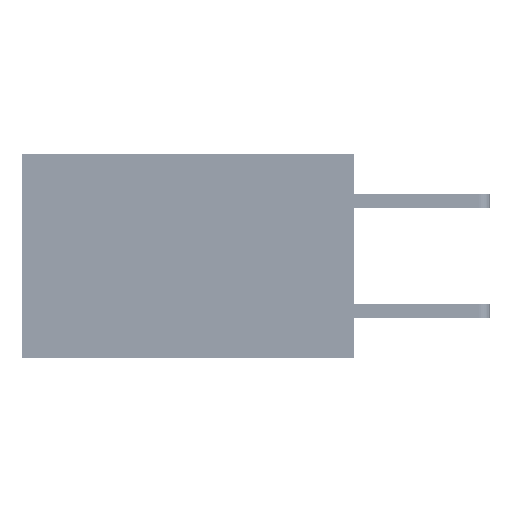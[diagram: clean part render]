
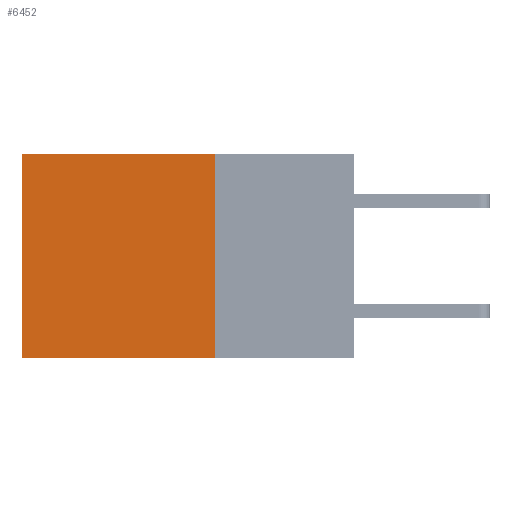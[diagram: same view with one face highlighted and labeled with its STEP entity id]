
A CAD part, left-side view. The second image highlights one B-rep face of the part: STEP entity #6452.
In plain terms, the highlighted planar face has unit normal (-1, 0, 0).
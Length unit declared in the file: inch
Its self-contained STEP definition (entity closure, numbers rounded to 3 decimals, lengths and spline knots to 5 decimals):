
#1216 = DIRECTION ( 'NONE',  ( 0., 0., -1. ) ) ;
#2729 = CARTESIAN_POINT ( 'NONE',  ( 0.2875, 0.25, -0.37 ) ) ;
#2798 = ORIENTED_EDGE ( 'NONE', *, *, #7453, .T. ) ;
#2869 = DIRECTION ( 'NONE',  ( 0., 1., 0. ) ) ;
#5285 = ORIENTED_EDGE ( 'NONE', *, *, #21799, .T. ) ;
#6452 = ADVANCED_FACE ( 'NONE', ( #37679 ), #11612, .F. ) ;
#7200 = VERTEX_POINT ( 'NONE', #37165 ) ;
#7284 = AXIS2_PLACEMENT_3D ( 'NONE', #11478, #27236, #24142 ) ;
#7453 = EDGE_CURVE ( 'NONE', #7200, #17033, #25143, .T. ) ;
#8992 = CARTESIAN_POINT ( 'NONE',  ( 0.2875, 0.6, 0. ) ) ;
#9237 = CARTESIAN_POINT ( 'NONE',  ( 0.2875, 0.25, -0.37 ) ) ;
#9628 = VECTOR ( 'NONE', #20769, 39.37008 ) ;
#10215 = VECTOR ( 'NONE', #2869, 39.37008 ) ;
#11478 = CARTESIAN_POINT ( 'NONE',  ( 0.2875, 0.25, 0. ) ) ;
#11612 = PLANE ( 'NONE',  #7284 ) ;
#14807 = VECTOR ( 'NONE', #26181, 39.37008 ) ;
#15288 = EDGE_CURVE ( 'NONE', #7200, #36131, #28277, .T. ) ;
#17033 = VERTEX_POINT ( 'NONE', #8992 ) ;
#20694 = CARTESIAN_POINT ( 'NONE',  ( 0.2875, 0.6, -0.37 ) ) ;
#20769 = DIRECTION ( 'NONE',  ( 0., 1., 0. ) ) ;
#20928 = ORIENTED_EDGE ( 'NONE', *, *, #15288, .F. ) ;
#20970 = EDGE_LOOP ( 'NONE', ( #5285, #35412, #20928, #2798 ) ) ;
#21799 = EDGE_CURVE ( 'NONE', #17033, #30639, #35271, .T. ) ;
#24142 = DIRECTION ( 'NONE',  ( 0., 0., -1. ) ) ;
#25143 = LINE ( 'NONE', #36661, #9628 ) ;
#26181 = DIRECTION ( 'NONE',  ( 0., 0., -1. ) ) ;
#27236 = DIRECTION ( 'NONE',  ( 1., 0., 0. ) ) ;
#28277 = LINE ( 'NONE', #29277, #14807 ) ;
#28812 = VECTOR ( 'NONE', #1216, 39.37008 ) ;
#29277 = CARTESIAN_POINT ( 'NONE',  ( 0.2875, 0.25, 0. ) ) ;
#30639 = VERTEX_POINT ( 'NONE', #20694 ) ;
#30764 = EDGE_CURVE ( 'NONE', #36131, #30639, #34166, .T. ) ;
#33286 = CARTESIAN_POINT ( 'NONE',  ( 0.2875, 0.6, 0. ) ) ;
#34166 = LINE ( 'NONE', #2729, #10215 ) ;
#35271 = LINE ( 'NONE', #33286, #28812 ) ;
#35412 = ORIENTED_EDGE ( 'NONE', *, *, #30764, .F. ) ;
#36131 = VERTEX_POINT ( 'NONE', #9237 ) ;
#36661 = CARTESIAN_POINT ( 'NONE',  ( 0.2875, 0.25, 0. ) ) ;
#37165 = CARTESIAN_POINT ( 'NONE',  ( 0.2875, 0.25, 0. ) ) ;
#37679 = FACE_OUTER_BOUND ( 'NONE', #20970, .T. ) ;
